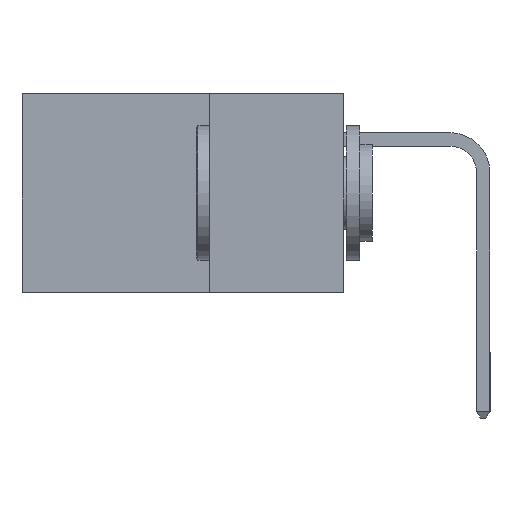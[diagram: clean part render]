
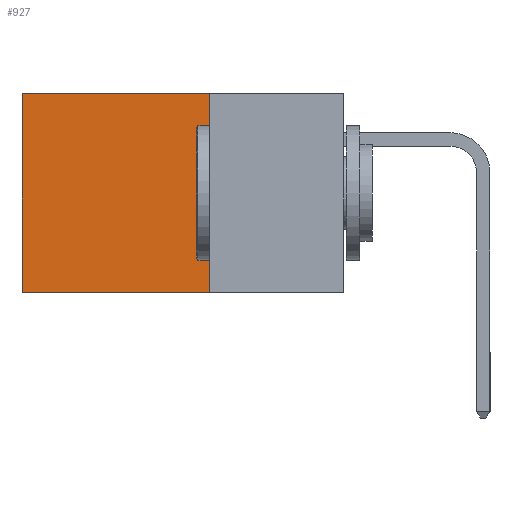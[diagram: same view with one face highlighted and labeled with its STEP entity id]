
A CAD part, left-side view. The second image highlights one B-rep face of the part: STEP entity #927.
In plain terms, the highlighted planar face has unit normal (-1, 0, 0).
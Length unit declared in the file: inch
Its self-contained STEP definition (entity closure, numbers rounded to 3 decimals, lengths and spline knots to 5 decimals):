
#81 = FACE_OUTER_BOUND ( 'NONE', #4587, .T. ) ;
#111 = DIRECTION ( 'NONE',  ( 0., 1., 0. ) ) ;
#552 = DIRECTION ( 'NONE',  ( 0., 0., -1. ) ) ;
#927 = ADVANCED_FACE ( 'NONE', ( #81 ), #5488, .F. ) ;
#1102 = CARTESIAN_POINT ( 'NONE',  ( 0.2615, 0.25, -0.37 ) ) ;
#1563 = LINE ( 'NONE', #3269, #4560 ) ;
#1796 = LINE ( 'NONE', #8597, #4843 ) ;
#1859 = VERTEX_POINT ( 'NONE', #9690 ) ;
#2084 = VECTOR ( 'NONE', #8807, 39.37008 ) ;
#2581 = EDGE_CURVE ( 'NONE', #1859, #10921, #1796, .T. ) ;
#2776 = CARTESIAN_POINT ( 'NONE',  ( 0.2615, 0.25, -0.37 ) ) ;
#3269 = CARTESIAN_POINT ( 'NONE',  ( 0.2615, 0.25, -0.37 ) ) ;
#3515 = DIRECTION ( 'NONE',  ( 1., 0., 0. ) ) ;
#3648 = CARTESIAN_POINT ( 'NONE',  ( 0.2615, 0.6, -0.37 ) ) ;
#3997 = EDGE_CURVE ( 'NONE', #1859, #4674, #1563, .T. ) ;
#4178 = VERTEX_POINT ( 'NONE', #3648 ) ;
#4560 = VECTOR ( 'NONE', #10089, 39.37008 ) ;
#4587 = EDGE_LOOP ( 'NONE', ( #8737, #7790, #8728, #6465 ) ) ;
#4674 = VERTEX_POINT ( 'NONE', #1102 ) ;
#4725 = DIRECTION ( 'NONE',  ( 0., 0., -1. ) ) ;
#4843 = VECTOR ( 'NONE', #111, 39.37008 ) ;
#5427 = CARTESIAN_POINT ( 'NONE',  ( 0.2615, 0.25, -0.37 ) ) ;
#5488 = PLANE ( 'NONE',  #6946 ) ;
#5972 = EDGE_CURVE ( 'NONE', #4674, #4178, #9581, .T. ) ;
#6465 = ORIENTED_EDGE ( 'NONE', *, *, #2581, .T. ) ;
#6946 = AXIS2_PLACEMENT_3D ( 'NONE', #5427, #3515, #4725 ) ;
#7030 = CARTESIAN_POINT ( 'NONE',  ( 0.2615, 0.6, -0.37 ) ) ;
#7148 = LINE ( 'NONE', #7030, #7276 ) ;
#7276 = VECTOR ( 'NONE', #552, 39.37008 ) ;
#7790 = ORIENTED_EDGE ( 'NONE', *, *, #5972, .F. ) ;
#8003 = EDGE_CURVE ( 'NONE', #10921, #4178, #7148, .T. ) ;
#8597 = CARTESIAN_POINT ( 'NONE',  ( 0.2615, 0.25, 0. ) ) ;
#8728 = ORIENTED_EDGE ( 'NONE', *, *, #3997, .F. ) ;
#8737 = ORIENTED_EDGE ( 'NONE', *, *, #8003, .T. ) ;
#8807 = DIRECTION ( 'NONE',  ( 0., 1., 0. ) ) ;
#9581 = LINE ( 'NONE', #2776, #2084 ) ;
#9690 = CARTESIAN_POINT ( 'NONE',  ( 0.2615, 0.25, 0. ) ) ;
#10089 = DIRECTION ( 'NONE',  ( 0., 0., -1. ) ) ;
#10184 = CARTESIAN_POINT ( 'NONE',  ( 0.2615, 0.6, 0. ) ) ;
#10921 = VERTEX_POINT ( 'NONE', #10184 ) ;
